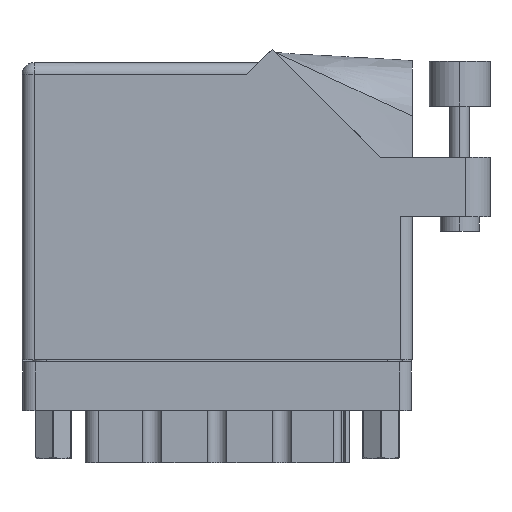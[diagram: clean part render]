
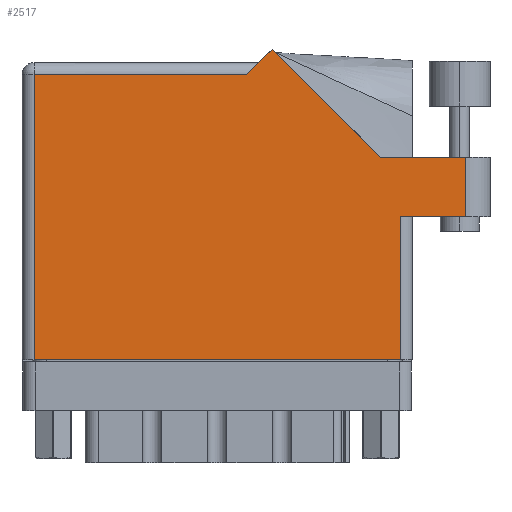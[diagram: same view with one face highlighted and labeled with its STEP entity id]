
A CAD part, front view. The second image highlights one B-rep face of the part: STEP entity #2517.
In plain terms, the highlighted face is planar.
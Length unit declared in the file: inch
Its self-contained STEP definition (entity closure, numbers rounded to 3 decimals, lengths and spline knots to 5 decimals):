
#251 = ORIENTED_EDGE ( 'NONE', *, *, #13670, .T. ) ;
#2061 = VECTOR ( 'NONE', #12759, 39.37008 ) ;
#2517 = ADVANCED_FACE ( 'NONE', ( #28075 ), #19789, .F. ) ;
#2904 = LINE ( 'NONE', #24843, #32363 ) ;
#3095 = EDGE_CURVE ( 'NONE', #29896, #22536, #44823, .T. ) ;
#4515 = CARTESIAN_POINT ( 'NONE',  ( 1.28771, 1.60071, 0. ) ) ;
#5374 = CARTESIAN_POINT ( 'NONE',  ( 1.948, 0., 0. ) ) ;
#9179 = ORIENTED_EDGE ( 'NONE', *, *, #10417, .T. ) ;
#9352 = EDGE_CURVE ( 'NONE', #13910, #29896, #10643, .T. ) ;
#9967 = ORIENTED_EDGE ( 'NONE', *, *, #3095, .T. ) ;
#10417 = EDGE_CURVE ( 'NONE', #27208, #11570, #18962, .T. ) ;
#10643 = LINE ( 'NONE', #36321, #24515 ) ;
#10662 = ORIENTED_EDGE ( 'NONE', *, *, #37327, .T. ) ;
#11570 = VERTEX_POINT ( 'NONE', #26476 ) ;
#11732 = ORIENTED_EDGE ( 'NONE', *, *, #15338, .T. ) ;
#12111 = VECTOR ( 'NONE', #41991, 39.37008 ) ;
#12346 = VECTOR ( 'NONE', #44444, 39.37008 ) ;
#12548 = DIRECTION ( 'NONE',  ( 0., 0., -1. ) ) ;
#12759 = DIRECTION ( 'NONE',  ( 1., 0., 0. ) ) ;
#13670 = EDGE_CURVE ( 'NONE', #47382, #13910, #33742, .T. ) ;
#13910 = VERTEX_POINT ( 'NONE', #24317 ) ;
#14429 = VERTEX_POINT ( 'NONE', #30656 ) ;
#15338 = EDGE_CURVE ( 'NONE', #14429, #35171, #26162, .T. ) ;
#15693 = LINE ( 'NONE', #21931, #16285 ) ;
#16285 = VECTOR ( 'NONE', #44802, 39.37008 ) ;
#16545 = VECTOR ( 'NONE', #32424, 39.37008 ) ;
#17873 = LINE ( 'NONE', #38228, #22693 ) ;
#18962 = LINE ( 'NONE', #32991, #12346 ) ;
#18997 = CARTESIAN_POINT ( 'NONE',  ( 1.948, 0.737, 0. ) ) ;
#19789 = PLANE ( 'NONE',  #37509 ) ;
#20172 = CARTESIAN_POINT ( 'NONE',  ( 0., 0., 0. ) ) ;
#21862 = CARTESIAN_POINT ( 'NONE',  ( 0.062, 1.468, 0. ) ) ;
#21931 = CARTESIAN_POINT ( 'NONE',  ( 1.948, 0.737, 0. ) ) ;
#22045 = CARTESIAN_POINT ( 'NONE',  ( 1.84442, 1.044, 0. ) ) ;
#22439 = EDGE_CURVE ( 'NONE', #43576, #14429, #49718, .T. ) ;
#22536 = VERTEX_POINT ( 'NONE', #22045 ) ;
#22575 = VECTOR ( 'NONE', #48488, 39.37008 ) ;
#22653 = CARTESIAN_POINT ( 'NONE',  ( 2.01, 0.737, 0. ) ) ;
#22693 = VECTOR ( 'NONE', #42407, 39.37008 ) ;
#24317 = CARTESIAN_POINT ( 'NONE',  ( 2.285, 0.737, 0. ) ) ;
#24515 = VECTOR ( 'NONE', #36824, 39.37008 ) ;
#24568 = ORIENTED_EDGE ( 'NONE', *, *, #43080, .T. ) ;
#24843 = CARTESIAN_POINT ( 'NONE',  ( 0., 1.468, 0. ) ) ;
#26162 = LINE ( 'NONE', #20172, #2061 ) ;
#26476 = CARTESIAN_POINT ( 'NONE',  ( 1.155, 1.468, 0. ) ) ;
#27208 = VERTEX_POINT ( 'NONE', #4515 ) ;
#27845 = CARTESIAN_POINT ( 'NONE',  ( 2.285, 1.044, 0. ) ) ;
#28075 = FACE_OUTER_BOUND ( 'NONE', #30280, .T. ) ;
#29896 = VERTEX_POINT ( 'NONE', #27845 ) ;
#30280 = EDGE_LOOP ( 'NONE', ( #251, #49643, #9967, #24568, #9179, #10662, #45551, #11732, #47854 ) ) ;
#30656 = CARTESIAN_POINT ( 'NONE',  ( 0.062, 0., 0. ) ) ;
#31369 = CARTESIAN_POINT ( 'NONE',  ( 0., 1.53, 0. ) ) ;
#32363 = VECTOR ( 'NONE', #40177, 39.37008 ) ;
#32424 = DIRECTION ( 'NONE',  ( -1., 0., 0. ) ) ;
#32991 = CARTESIAN_POINT ( 'NONE',  ( 1.217, 1.53, 0. ) ) ;
#33447 = CARTESIAN_POINT ( 'NONE',  ( 0.062, 0., 0. ) ) ;
#33742 = LINE ( 'NONE', #22653, #12111 ) ;
#35042 = DIRECTION ( 'NONE',  ( -1., 0., 0. ) ) ;
#35171 = VERTEX_POINT ( 'NONE', #5374 ) ;
#36321 = CARTESIAN_POINT ( 'NONE',  ( 2.285, 1.044, 0. ) ) ;
#36824 = DIRECTION ( 'NONE',  ( 0., 1., 0. ) ) ;
#37327 = EDGE_CURVE ( 'NONE', #11570, #43576, #2904, .T. ) ;
#37509 = AXIS2_PLACEMENT_3D ( 'NONE', #31369, #12548, #35042 ) ;
#38228 = CARTESIAN_POINT ( 'NONE',  ( 1.84442, 1.044, 0. ) ) ;
#40177 = DIRECTION ( 'NONE',  ( -1., 0., 0. ) ) ;
#41991 = DIRECTION ( 'NONE',  ( 1., 0., 0. ) ) ;
#42407 = DIRECTION ( 'NONE',  ( -0.707, 0.707, 0. ) ) ;
#43080 = EDGE_CURVE ( 'NONE', #22536, #27208, #17873, .T. ) ;
#43381 = CARTESIAN_POINT ( 'NONE',  ( 2.41, 1.044, 0. ) ) ;
#43576 = VERTEX_POINT ( 'NONE', #21862 ) ;
#44444 = DIRECTION ( 'NONE',  ( -0.707, -0.707, 0. ) ) ;
#44802 = DIRECTION ( 'NONE',  ( 0., 1., 0. ) ) ;
#44823 = LINE ( 'NONE', #43381, #16545 ) ;
#45551 = ORIENTED_EDGE ( 'NONE', *, *, #22439, .T. ) ;
#47382 = VERTEX_POINT ( 'NONE', #18997 ) ;
#47854 = ORIENTED_EDGE ( 'NONE', *, *, #48331, .T. ) ;
#48331 = EDGE_CURVE ( 'NONE', #35171, #47382, #15693, .T. ) ;
#48488 = DIRECTION ( 'NONE',  ( 0., -1., 0. ) ) ;
#49643 = ORIENTED_EDGE ( 'NONE', *, *, #9352, .T. ) ;
#49718 = LINE ( 'NONE', #33447, #22575 ) ;
